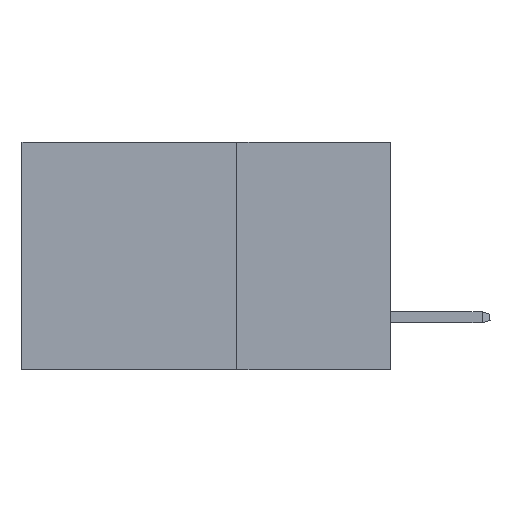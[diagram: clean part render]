
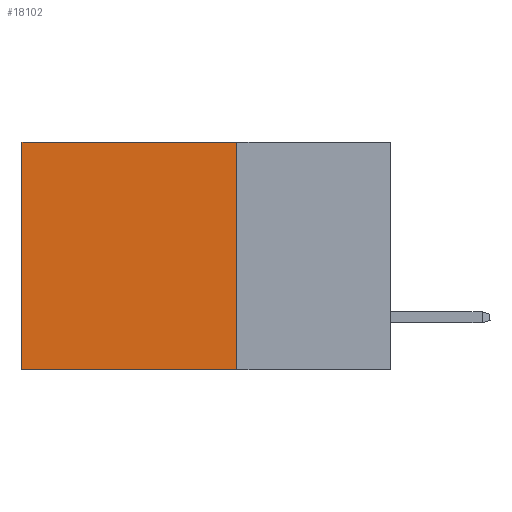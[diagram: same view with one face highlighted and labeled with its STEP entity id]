
A CAD part, left-side view. The second image highlights one B-rep face of the part: STEP entity #18102.
In plain terms, the highlighted planar face has unit normal (-1, 0, 0).
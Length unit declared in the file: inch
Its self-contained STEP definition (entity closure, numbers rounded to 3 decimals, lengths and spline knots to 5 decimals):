
#1110 = CARTESIAN_POINT ( 'NONE',  ( 0.2875, 0.25, -0.37 ) ) ;
#1696 = VERTEX_POINT ( 'NONE', #14051 ) ;
#2709 = DIRECTION ( 'NONE',  ( 0., 1., 0. ) ) ;
#3421 = ORIENTED_EDGE ( 'NONE', *, *, #18241, .F. ) ;
#3467 = ORIENTED_EDGE ( 'NONE', *, *, #22110, .T. ) ;
#3549 = ORIENTED_EDGE ( 'NONE', *, *, #11984, .T. ) ;
#4099 = AXIS2_PLACEMENT_3D ( 'NONE', #12360, #4829, #15449 ) ;
#4209 = ORIENTED_EDGE ( 'NONE', *, *, #17958, .F. ) ;
#4829 = DIRECTION ( 'NONE',  ( 1., 0., 0. ) ) ;
#5211 = DIRECTION ( 'NONE',  ( 0., 0., -1. ) ) ;
#5249 = CARTESIAN_POINT ( 'NONE',  ( 0.2875, 0.6, 0. ) ) ;
#5775 = LINE ( 'NONE', #1110, #14466 ) ;
#6119 = LINE ( 'NONE', #5249, #18846 ) ;
#6992 = DIRECTION ( 'NONE',  ( 0., 0., -1. ) ) ;
#7610 = CARTESIAN_POINT ( 'NONE',  ( 0.2875, 0.25, 0. ) ) ;
#9387 = DIRECTION ( 'NONE',  ( 0., 1., 0. ) ) ;
#9989 = CARTESIAN_POINT ( 'NONE',  ( 0.2875, 0.25, 0. ) ) ;
#11508 = VECTOR ( 'NONE', #5211, 39.37008 ) ;
#11984 = EDGE_CURVE ( 'NONE', #14205, #13355, #21556, .T. ) ;
#12073 = FACE_OUTER_BOUND ( 'NONE', #19368, .T. ) ;
#12360 = CARTESIAN_POINT ( 'NONE',  ( 0.2875, 0.25, 0. ) ) ;
#13110 = LINE ( 'NONE', #18933, #11508 ) ;
#13355 = VERTEX_POINT ( 'NONE', #21838 ) ;
#14051 = CARTESIAN_POINT ( 'NONE',  ( 0.2875, 0.25, -0.37 ) ) ;
#14205 = VERTEX_POINT ( 'NONE', #9989 ) ;
#14466 = VECTOR ( 'NONE', #2709, 39.37008 ) ;
#15279 = PLANE ( 'NONE',  #4099 ) ;
#15449 = DIRECTION ( 'NONE',  ( 0., 0., -1. ) ) ;
#16481 = VECTOR ( 'NONE', #9387, 39.37008 ) ;
#16912 = VERTEX_POINT ( 'NONE', #20785 ) ;
#17958 = EDGE_CURVE ( 'NONE', #1696, #16912, #5775, .T. ) ;
#18102 = ADVANCED_FACE ( 'NONE', ( #12073 ), #15279, .F. ) ;
#18241 = EDGE_CURVE ( 'NONE', #14205, #1696, #13110, .T. ) ;
#18846 = VECTOR ( 'NONE', #6992, 39.37008 ) ;
#18933 = CARTESIAN_POINT ( 'NONE',  ( 0.2875, 0.25, 0. ) ) ;
#19368 = EDGE_LOOP ( 'NONE', ( #3467, #4209, #3421, #3549 ) ) ;
#20785 = CARTESIAN_POINT ( 'NONE',  ( 0.2875, 0.6, -0.37 ) ) ;
#21556 = LINE ( 'NONE', #7610, #16481 ) ;
#21838 = CARTESIAN_POINT ( 'NONE',  ( 0.2875, 0.6, 0. ) ) ;
#22110 = EDGE_CURVE ( 'NONE', #13355, #16912, #6119, .T. ) ;
